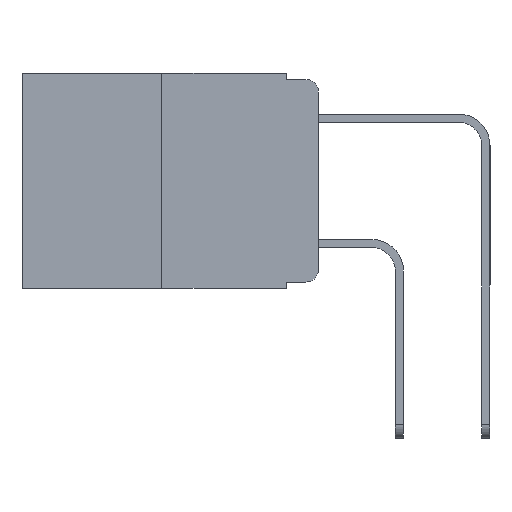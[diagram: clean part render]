
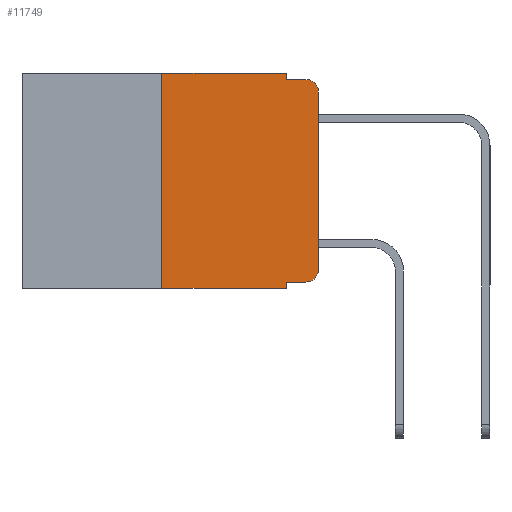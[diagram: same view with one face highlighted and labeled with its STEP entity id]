
A CAD part, left-side view. The second image highlights one B-rep face of the part: STEP entity #11749.
In plain terms, the highlighted planar face has unit normal (-1, 0, 0).
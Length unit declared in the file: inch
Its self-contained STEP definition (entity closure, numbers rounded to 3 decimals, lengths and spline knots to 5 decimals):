
#282 = VERTEX_POINT ( 'NONE', #16428 ) ;
#453 = VERTEX_POINT ( 'NONE', #5846 ) ;
#753 = EDGE_CURVE ( 'NONE', #282, #7922, #10956, .T. ) ;
#798 = DIRECTION ( 'NONE',  ( 0., 0., -1. ) ) ;
#1215 = EDGE_CURVE ( 'NONE', #7376, #10029, #14114, .T. ) ;
#1378 = ORIENTED_EDGE ( 'NONE', *, *, #15957, .T. ) ;
#1666 = CARTESIAN_POINT ( 'NONE',  ( 0., 0., -0.313 ) ) ;
#2258 = DIRECTION ( 'NONE',  ( 0., 0., -1. ) ) ;
#2578 = EDGE_CURVE ( 'NONE', #3643, #8583, #15363, .T. ) ;
#2760 = VECTOR ( 'NONE', #9903, 39.37008 ) ;
#3393 = VERTEX_POINT ( 'NONE', #17702 ) ;
#3473 = PLANE ( 'NONE',  #6755 ) ;
#3643 = VERTEX_POINT ( 'NONE', #7294 ) ;
#3729 = ORIENTED_EDGE ( 'NONE', *, *, #1215, .T. ) ;
#4245 = VECTOR ( 'NONE', #10910, 39.37008 ) ;
#4885 = DIRECTION ( 'NONE',  ( 0., 0., -1. ) ) ;
#5751 = CARTESIAN_POINT ( 'NONE',  ( 0., 0.051, 0. ) ) ;
#5846 = CARTESIAN_POINT ( 'NONE',  ( 0., 0.02, -0.01 ) ) ;
#5873 = CARTESIAN_POINT ( 'NONE',  ( 0., 0.473, -0.343 ) ) ;
#6289 = LINE ( 'NONE', #5751, #13159 ) ;
#6322 = VECTOR ( 'NONE', #8356, 39.37008 ) ;
#6388 = VERTEX_POINT ( 'NONE', #17600 ) ;
#6755 = AXIS2_PLACEMENT_3D ( 'NONE', #14487, #13142, #4885 ) ;
#6795 = VECTOR ( 'NONE', #9104, 39.37008 ) ;
#6937 = CARTESIAN_POINT ( 'NONE',  ( 0., 0.25, 0. ) ) ;
#7150 = AXIS2_PLACEMENT_3D ( 'NONE', #17490, #9344, #798 ) ;
#7266 = DIRECTION ( 'NONE',  ( 0., -1., 0. ) ) ;
#7294 = CARTESIAN_POINT ( 'NONE',  ( 0., 0.051, -0.333 ) ) ;
#7376 = VERTEX_POINT ( 'NONE', #1666 ) ;
#7419 = LINE ( 'NONE', #16711, #2760 ) ;
#7552 = CARTESIAN_POINT ( 'NONE',  ( 0., 0., -0.03 ) ) ;
#7622 = CARTESIAN_POINT ( 'NONE',  ( 0., 0.02, -0.03 ) ) ;
#7922 = VERTEX_POINT ( 'NONE', #8912 ) ;
#7953 = LINE ( 'NONE', #5873, #8370 ) ;
#8269 = EDGE_CURVE ( 'NONE', #6388, #282, #17258, .T. ) ;
#8356 = DIRECTION ( 'NONE',  ( 0., 0., 1. ) ) ;
#8370 = VECTOR ( 'NONE', #7266, 39.37008 ) ;
#8583 = VERTEX_POINT ( 'NONE', #14457 ) ;
#8839 = EDGE_LOOP ( 'NONE', ( #3729, #9626, #17964, #15879, #15299, #15516, #14057, #8935, #17893, #1378 ) ) ;
#8912 = CARTESIAN_POINT ( 'NONE',  ( 0., 0.051, 0. ) ) ;
#8935 = ORIENTED_EDGE ( 'NONE', *, *, #2578, .F. ) ;
#9013 = DIRECTION ( 'NONE',  ( 0., 0., -1. ) ) ;
#9104 = DIRECTION ( 'NONE',  ( 0., 0., 1. ) ) ;
#9202 = EDGE_CURVE ( 'NONE', #7922, #17224, #6289, .T. ) ;
#9344 = DIRECTION ( 'NONE',  ( -1., 0., 0. ) ) ;
#9626 = ORIENTED_EDGE ( 'NONE', *, *, #14703, .T. ) ;
#9821 = AXIS2_PLACEMENT_3D ( 'NONE', #7622, #17176, #9013 ) ;
#9903 = DIRECTION ( 'NONE',  ( 0., -1., 0. ) ) ;
#10029 = VERTEX_POINT ( 'NONE', #7552 ) ;
#10910 = DIRECTION ( 'NONE',  ( 0., -1., 0. ) ) ;
#10956 = LINE ( 'NONE', #13576, #17739 ) ;
#11047 = EDGE_CURVE ( 'NONE', #17224, #453, #15267, .T. ) ;
#11131 = CIRCLE ( 'NONE', #7150, 0.02 ) ;
#11725 = VECTOR ( 'NONE', #2258, 39.37008 ) ;
#11749 = ADVANCED_FACE ( 'NONE', ( #11819 ), #3473, .F. ) ;
#11819 = FACE_OUTER_BOUND ( 'NONE', #8839, .T. ) ;
#12050 = CARTESIAN_POINT ( 'NONE',  ( 0., 0.051, 0. ) ) ;
#12189 = CARTESIAN_POINT ( 'NONE',  ( 0., 0.051, -0.01 ) ) ;
#12209 = CARTESIAN_POINT ( 'NONE',  ( 0., 0.051, -0.01 ) ) ;
#12279 = DIRECTION ( 'NONE',  ( 0., -1., 0. ) ) ;
#13142 = DIRECTION ( 'NONE',  ( 1., 0., 0. ) ) ;
#13159 = VECTOR ( 'NONE', #18067, 39.37008 ) ;
#13195 = CARTESIAN_POINT ( 'NONE',  ( 0., 0., 0. ) ) ;
#13576 = CARTESIAN_POINT ( 'NONE',  ( 0., 0.473, 0. ) ) ;
#13921 = EDGE_CURVE ( 'NONE', #6388, #8583, #7953, .T. ) ;
#14057 = ORIENTED_EDGE ( 'NONE', *, *, #13921, .T. ) ;
#14114 = LINE ( 'NONE', #13195, #6795 ) ;
#14457 = CARTESIAN_POINT ( 'NONE',  ( 0., 0.051, -0.343 ) ) ;
#14487 = CARTESIAN_POINT ( 'NONE',  ( 0., 0.473, 0. ) ) ;
#14703 = EDGE_CURVE ( 'NONE', #10029, #453, #16488, .T. ) ;
#15267 = LINE ( 'NONE', #12209, #4245 ) ;
#15299 = ORIENTED_EDGE ( 'NONE', *, *, #753, .F. ) ;
#15363 = LINE ( 'NONE', #12050, #11725 ) ;
#15516 = ORIENTED_EDGE ( 'NONE', *, *, #8269, .F. ) ;
#15879 = ORIENTED_EDGE ( 'NONE', *, *, #9202, .F. ) ;
#15957 = EDGE_CURVE ( 'NONE', #3393, #7376, #11131, .T. ) ;
#16428 = CARTESIAN_POINT ( 'NONE',  ( 0., 0.25, 0. ) ) ;
#16488 = CIRCLE ( 'NONE', #9821, 0.02 ) ;
#16711 = CARTESIAN_POINT ( 'NONE',  ( 0., 0.051, -0.333 ) ) ;
#16850 = EDGE_CURVE ( 'NONE', #3643, #3393, #7419, .T. ) ;
#17176 = DIRECTION ( 'NONE',  ( -1., 0., 0. ) ) ;
#17224 = VERTEX_POINT ( 'NONE', #12189 ) ;
#17258 = LINE ( 'NONE', #6937, #6322 ) ;
#17490 = CARTESIAN_POINT ( 'NONE',  ( 0., 0.02, -0.313 ) ) ;
#17600 = CARTESIAN_POINT ( 'NONE',  ( 0., 0.25, -0.343 ) ) ;
#17702 = CARTESIAN_POINT ( 'NONE',  ( 0., 0.02, -0.333 ) ) ;
#17739 = VECTOR ( 'NONE', #12279, 39.37008 ) ;
#17893 = ORIENTED_EDGE ( 'NONE', *, *, #16850, .T. ) ;
#17964 = ORIENTED_EDGE ( 'NONE', *, *, #11047, .F. ) ;
#18067 = DIRECTION ( 'NONE',  ( 0., 0., -1. ) ) ;
